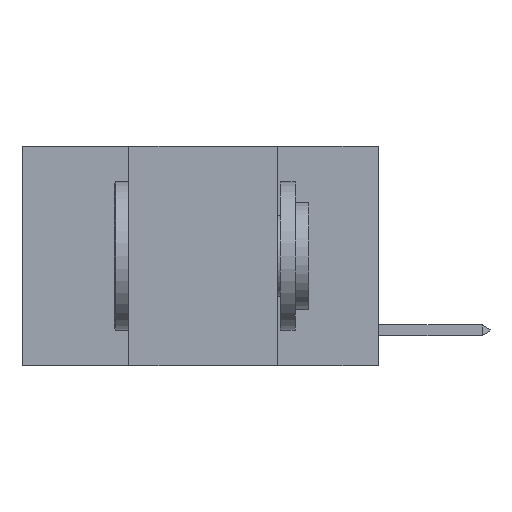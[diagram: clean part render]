
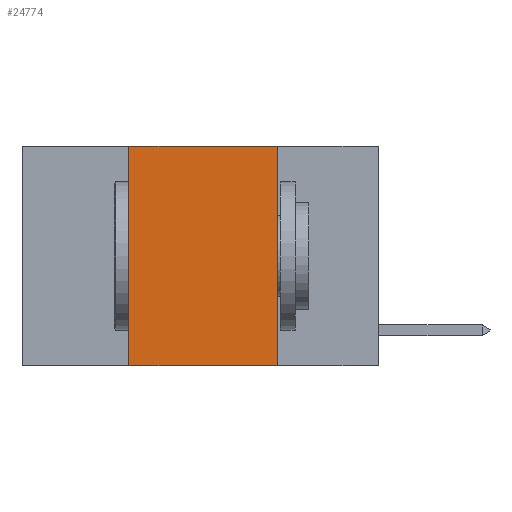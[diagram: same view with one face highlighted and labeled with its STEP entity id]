
A CAD part, left-side view. The second image highlights one B-rep face of the part: STEP entity #24774.
In plain terms, the highlighted planar face has unit normal (-1, 0, 0).
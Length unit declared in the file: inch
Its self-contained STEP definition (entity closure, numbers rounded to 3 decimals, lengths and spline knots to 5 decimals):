
#222 = ORIENTED_EDGE ( 'NONE', *, *, #26893, .F. ) ;
#1083 = ORIENTED_EDGE ( 'NONE', *, *, #19406, .T. ) ;
#1394 = CARTESIAN_POINT ( 'NONE',  ( 0., 0.42, 0. ) ) ;
#1919 = LINE ( 'NONE', #1394, #23402 ) ;
#2859 = LINE ( 'NONE', #11589, #16990 ) ;
#4246 = VECTOR ( 'NONE', #16793, 39.37008 ) ;
#4669 = FACE_OUTER_BOUND ( 'NONE', #27062, .T. ) ;
#4890 = LINE ( 'NONE', #22538, #7989 ) ;
#7350 = EDGE_CURVE ( 'NONE', #24448, #14233, #1919, .T. ) ;
#7989 = VECTOR ( 'NONE', #20654, 39.37008 ) ;
#8163 = CARTESIAN_POINT ( 'NONE',  ( 0., 0.6, 0. ) ) ;
#8953 = CARTESIAN_POINT ( 'NONE',  ( 0., 0.17, 0. ) ) ;
#10702 = VERTEX_POINT ( 'NONE', #8953 ) ;
#11471 = ORIENTED_EDGE ( 'NONE', *, *, #7350, .F. ) ;
#11589 = CARTESIAN_POINT ( 'NONE',  ( 0., 0.6, -0.37 ) ) ;
#11675 = DIRECTION ( 'NONE',  ( 0., 0., -1. ) ) ;
#11725 = CARTESIAN_POINT ( 'NONE',  ( 0., 0.42, 0. ) ) ;
#11852 = CARTESIAN_POINT ( 'NONE',  ( 0., 0.42, -0.37 ) ) ;
#13695 = PLANE ( 'NONE',  #17149 ) ;
#14233 = VERTEX_POINT ( 'NONE', #11725 ) ;
#14992 = CARTESIAN_POINT ( 'NONE',  ( 0., 0.17, -0.37 ) ) ;
#15426 = CARTESIAN_POINT ( 'NONE',  ( 0., 0.6, 0. ) ) ;
#16364 = LINE ( 'NONE', #8163, #4246 ) ;
#16793 = DIRECTION ( 'NONE',  ( 0., -1., 0. ) ) ;
#16990 = VECTOR ( 'NONE', #20619, 39.37008 ) ;
#17149 = AXIS2_PLACEMENT_3D ( 'NONE', #15426, #26767, #11675 ) ;
#17266 = DIRECTION ( 'NONE',  ( 0., 0., 1. ) ) ;
#19406 = EDGE_CURVE ( 'NONE', #24448, #21489, #2859, .T. ) ;
#20619 = DIRECTION ( 'NONE',  ( 0., -1., 0. ) ) ;
#20654 = DIRECTION ( 'NONE',  ( 0., 0., -1. ) ) ;
#21489 = VERTEX_POINT ( 'NONE', #14992 ) ;
#22354 = EDGE_CURVE ( 'NONE', #14233, #10702, #16364, .T. ) ;
#22538 = CARTESIAN_POINT ( 'NONE',  ( 0., 0.17, 0. ) ) ;
#23402 = VECTOR ( 'NONE', #17266, 39.37008 ) ;
#24448 = VERTEX_POINT ( 'NONE', #11852 ) ;
#24774 = ADVANCED_FACE ( 'NONE', ( #4669 ), #13695, .F. ) ;
#25545 = ORIENTED_EDGE ( 'NONE', *, *, #22354, .F. ) ;
#26767 = DIRECTION ( 'NONE',  ( 1., 0., 0. ) ) ;
#26893 = EDGE_CURVE ( 'NONE', #10702, #21489, #4890, .T. ) ;
#27062 = EDGE_LOOP ( 'NONE', ( #222, #25545, #11471, #1083 ) ) ;
